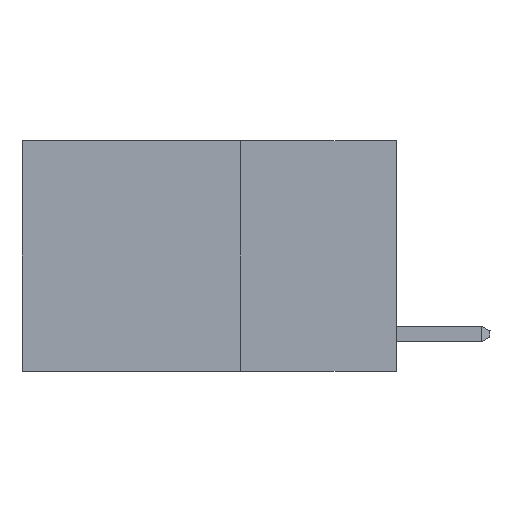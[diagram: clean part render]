
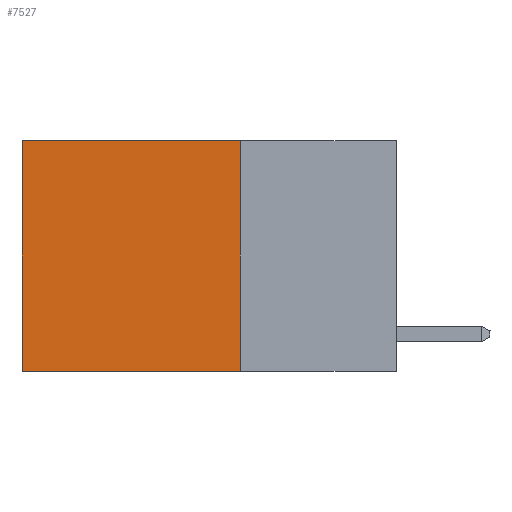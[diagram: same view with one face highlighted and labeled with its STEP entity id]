
A CAD part, left-side view. The second image highlights one B-rep face of the part: STEP entity #7527.
In plain terms, the highlighted planar face has unit normal (-1, 0, 0).
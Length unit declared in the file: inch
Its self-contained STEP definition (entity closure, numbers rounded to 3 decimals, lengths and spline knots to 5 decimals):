
#370 = LINE ( 'NONE', #20704, #14877 ) ;
#2835 = CARTESIAN_POINT ( 'NONE',  ( 0.2625, 0.25, 0. ) ) ;
#3059 = VECTOR ( 'NONE', #9154, 39.37008 ) ;
#3094 = LINE ( 'NONE', #5465, #13924 ) ;
#3477 = CARTESIAN_POINT ( 'NONE',  ( 0.2625, 0.25, -0.37 ) ) ;
#4440 = LINE ( 'NONE', #18078, #6011 ) ;
#4766 = DIRECTION ( 'NONE',  ( 0., 0., -1. ) ) ;
#5465 = CARTESIAN_POINT ( 'NONE',  ( 0.2625, 0.6, 0. ) ) ;
#5990 = EDGE_CURVE ( 'NONE', #22171, #19270, #370, .T. ) ;
#6011 = VECTOR ( 'NONE', #21679, 39.37008 ) ;
#6122 = FACE_OUTER_BOUND ( 'NONE', #18470, .T. ) ;
#6697 = EDGE_CURVE ( 'NONE', #24516, #12439, #3094, .T. ) ;
#7527 = ADVANCED_FACE ( 'NONE', ( #6122 ), #20492, .F. ) ;
#8640 = LINE ( 'NONE', #25036, #3059 ) ;
#9154 = DIRECTION ( 'NONE',  ( 0., 1., 0. ) ) ;
#9301 = ORIENTED_EDGE ( 'NONE', *, *, #5990, .F. ) ;
#10751 = ORIENTED_EDGE ( 'NONE', *, *, #10770, .T. ) ;
#10770 = EDGE_CURVE ( 'NONE', #22171, #24516, #4440, .T. ) ;
#12439 = VERTEX_POINT ( 'NONE', #16800 ) ;
#12653 = ORIENTED_EDGE ( 'NONE', *, *, #18489, .F. ) ;
#13924 = VECTOR ( 'NONE', #24994, 39.37008 ) ;
#14877 = VECTOR ( 'NONE', #4766, 39.37008 ) ;
#15446 = CARTESIAN_POINT ( 'NONE',  ( 0.2625, 0.6, 0. ) ) ;
#16800 = CARTESIAN_POINT ( 'NONE',  ( 0.2625, 0.6, -0.37 ) ) ;
#18078 = CARTESIAN_POINT ( 'NONE',  ( 0.2625, 0.25, 0. ) ) ;
#18470 = EDGE_LOOP ( 'NONE', ( #25018, #12653, #9301, #10751 ) ) ;
#18489 = EDGE_CURVE ( 'NONE', #19270, #12439, #8640, .T. ) ;
#19270 = VERTEX_POINT ( 'NONE', #3477 ) ;
#20404 = DIRECTION ( 'NONE',  ( 1., 0., 0. ) ) ;
#20492 = PLANE ( 'NONE',  #25144 ) ;
#20500 = CARTESIAN_POINT ( 'NONE',  ( 0.2625, 0.25, 0. ) ) ;
#20704 = CARTESIAN_POINT ( 'NONE',  ( 0.2625, 0.25, 0. ) ) ;
#21679 = DIRECTION ( 'NONE',  ( 0., 1., 0. ) ) ;
#22171 = VERTEX_POINT ( 'NONE', #20500 ) ;
#24413 = DIRECTION ( 'NONE',  ( 0., 0., -1. ) ) ;
#24516 = VERTEX_POINT ( 'NONE', #15446 ) ;
#24994 = DIRECTION ( 'NONE',  ( 0., 0., -1. ) ) ;
#25018 = ORIENTED_EDGE ( 'NONE', *, *, #6697, .T. ) ;
#25036 = CARTESIAN_POINT ( 'NONE',  ( 0.2625, 0.25, -0.37 ) ) ;
#25144 = AXIS2_PLACEMENT_3D ( 'NONE', #2835, #20404, #24413 ) ;
